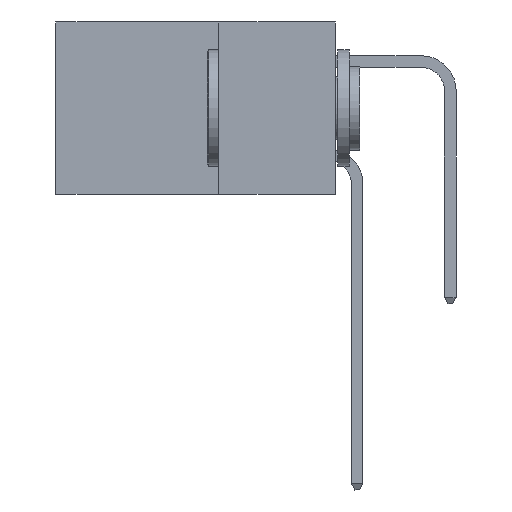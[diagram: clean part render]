
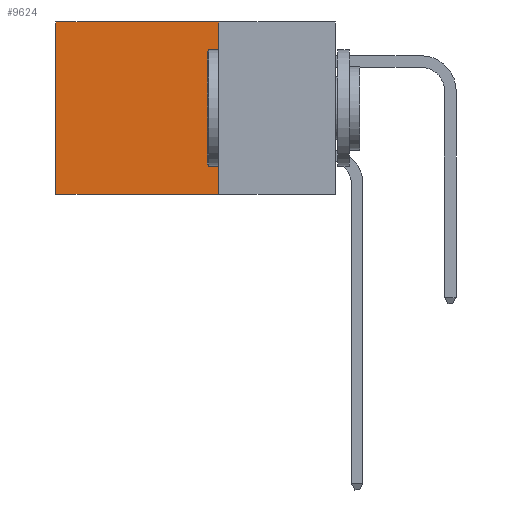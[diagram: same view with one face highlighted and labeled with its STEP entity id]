
A CAD part, left-side view. The second image highlights one B-rep face of the part: STEP entity #9624.
In plain terms, the highlighted planar face has unit normal (-1, 0, 0).
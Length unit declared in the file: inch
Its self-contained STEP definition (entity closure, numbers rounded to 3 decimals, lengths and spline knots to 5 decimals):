
#323 = CARTESIAN_POINT ( 'NONE',  ( 0.2875, 0.6, 0. ) ) ;
#1156 = CARTESIAN_POINT ( 'NONE',  ( 0.2875, 0.25, -0.37 ) ) ;
#2752 = EDGE_CURVE ( 'NONE', #11272, #16268, #5116, .T. ) ;
#2825 = VERTEX_POINT ( 'NONE', #25462 ) ;
#3435 = EDGE_CURVE ( 'NONE', #2825, #11272, #8565, .T. ) ;
#5116 = LINE ( 'NONE', #323, #13627 ) ;
#5155 = CARTESIAN_POINT ( 'NONE',  ( 0.2875, 0.25, 0. ) ) ;
#5312 = ORIENTED_EDGE ( 'NONE', *, *, #3435, .T. ) ;
#8489 = AXIS2_PLACEMENT_3D ( 'NONE', #5155, #22501, #27462 ) ;
#8565 = LINE ( 'NONE', #13243, #12425 ) ;
#9195 = EDGE_CURVE ( 'NONE', #2825, #21500, #16342, .T. ) ;
#9624 = ADVANCED_FACE ( 'NONE', ( #22808 ), #25290, .F. ) ;
#9768 = LINE ( 'NONE', #20038, #18305 ) ;
#10543 = ORIENTED_EDGE ( 'NONE', *, *, #9195, .F. ) ;
#10889 = ORIENTED_EDGE ( 'NONE', *, *, #21228, .F. ) ;
#11272 = VERTEX_POINT ( 'NONE', #20105 ) ;
#12075 = VECTOR ( 'NONE', #14647, 39.37008 ) ;
#12425 = VECTOR ( 'NONE', #25705, 39.37008 ) ;
#12568 = DIRECTION ( 'NONE',  ( 0., 0., -1. ) ) ;
#13243 = CARTESIAN_POINT ( 'NONE',  ( 0.2875, 0.25, 0. ) ) ;
#13513 = ORIENTED_EDGE ( 'NONE', *, *, #2752, .T. ) ;
#13627 = VECTOR ( 'NONE', #12568, 39.37008 ) ;
#14624 = DIRECTION ( 'NONE',  ( 0., 1., 0. ) ) ;
#14647 = DIRECTION ( 'NONE',  ( 0., 0., -1. ) ) ;
#16268 = VERTEX_POINT ( 'NONE', #25346 ) ;
#16342 = LINE ( 'NONE', #28857, #12075 ) ;
#17352 = EDGE_LOOP ( 'NONE', ( #13513, #10889, #10543, #5312 ) ) ;
#18305 = VECTOR ( 'NONE', #14624, 39.37008 ) ;
#20038 = CARTESIAN_POINT ( 'NONE',  ( 0.2875, 0.25, -0.37 ) ) ;
#20105 = CARTESIAN_POINT ( 'NONE',  ( 0.2875, 0.6, 0. ) ) ;
#21228 = EDGE_CURVE ( 'NONE', #21500, #16268, #9768, .T. ) ;
#21500 = VERTEX_POINT ( 'NONE', #1156 ) ;
#22501 = DIRECTION ( 'NONE',  ( 1., 0., 0. ) ) ;
#22808 = FACE_OUTER_BOUND ( 'NONE', #17352, .T. ) ;
#25290 = PLANE ( 'NONE',  #8489 ) ;
#25346 = CARTESIAN_POINT ( 'NONE',  ( 0.2875, 0.6, -0.37 ) ) ;
#25462 = CARTESIAN_POINT ( 'NONE',  ( 0.2875, 0.25, 0. ) ) ;
#25705 = DIRECTION ( 'NONE',  ( 0., 1., 0. ) ) ;
#27462 = DIRECTION ( 'NONE',  ( 0., 0., -1. ) ) ;
#28857 = CARTESIAN_POINT ( 'NONE',  ( 0.2875, 0.25, 0. ) ) ;
